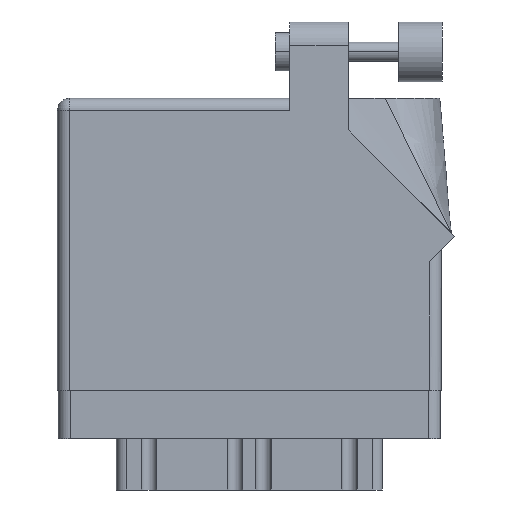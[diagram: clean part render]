
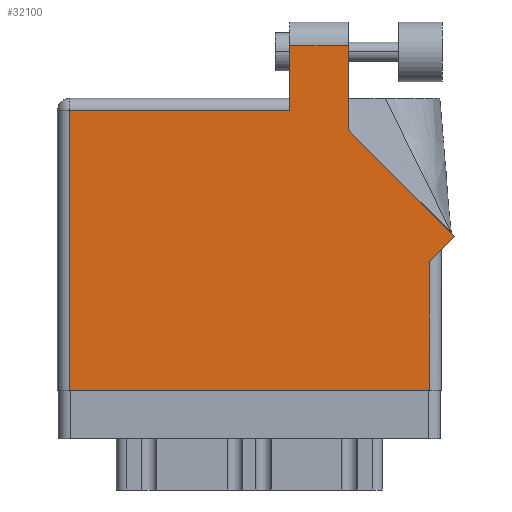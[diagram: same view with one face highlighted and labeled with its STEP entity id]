
A CAD part, front view. The second image highlights one B-rep face of the part: STEP entity #32100.
In plain terms, the highlighted face is planar.
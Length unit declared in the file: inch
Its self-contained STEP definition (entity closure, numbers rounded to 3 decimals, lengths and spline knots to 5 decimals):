
#353 = LINE ( 'NONE', #11561, #33160 ) ;
#774 = DIRECTION ( 'NONE',  ( -0.707, 0.707, 0. ) ) ;
#1603 = ORIENTED_EDGE ( 'NONE', *, *, #16011, .T. ) ;
#1677 = DIRECTION ( 'NONE',  ( 0., -1., 0. ) ) ;
#3643 = VECTOR ( 'NONE', #8445, 39.37008 ) ;
#3685 = DIRECTION ( 'NONE',  ( -1., 0., 0. ) ) ;
#4979 = LINE ( 'NONE', #26040, #32071 ) ;
#5489 = ORIENTED_EDGE ( 'NONE', *, *, #28860, .T. ) ;
#5757 = EDGE_CURVE ( 'NONE', #19924, #21574, #16168, .T. ) ;
#6481 = DIRECTION ( 'NONE',  ( 0., 0., -1. ) ) ;
#7013 = VERTEX_POINT ( 'NONE', #24255 ) ;
#7125 = ORIENTED_EDGE ( 'NONE', *, *, #5757, .T. ) ;
#7313 = VECTOR ( 'NONE', #7698, 39.37008 ) ;
#7698 = DIRECTION ( 'NONE',  ( 1., 0., 0. ) ) ;
#7923 = CARTESIAN_POINT ( 'NONE',  ( 0.062, 1.468, 0. ) ) ;
#8445 = DIRECTION ( 'NONE',  ( 0., 1., 0. ) ) ;
#10017 = ORIENTED_EDGE ( 'NONE', *, *, #15736, .T. ) ;
#11110 = CARTESIAN_POINT ( 'NONE',  ( 2.08071, 0.80771, 0. ) ) ;
#11286 = EDGE_CURVE ( 'NONE', #31697, #19924, #23322, .T. ) ;
#11561 = CARTESIAN_POINT ( 'NONE',  ( 1.217, 1.805, 0. ) ) ;
#11935 = CARTESIAN_POINT ( 'NONE',  ( 1.948, 0., 0. ) ) ;
#12372 = CARTESIAN_POINT ( 'NONE',  ( 2.01, 0.737, 0. ) ) ;
#12981 = VECTOR ( 'NONE', #1677, 39.37008 ) ;
#13047 = CARTESIAN_POINT ( 'NONE',  ( 1.524, 1.805, 0. ) ) ;
#13271 = VERTEX_POINT ( 'NONE', #7923 ) ;
#14476 = DIRECTION ( 'NONE',  ( 0.707, 0.707, 0. ) ) ;
#14502 = EDGE_CURVE ( 'NONE', #21574, #20996, #17464, .T. ) ;
#14668 = CARTESIAN_POINT ( 'NONE',  ( 1.217, 1.53, 0. ) ) ;
#15683 = DIRECTION ( 'NONE',  ( 0., 1., 0. ) ) ;
#15736 = EDGE_CURVE ( 'NONE', #21581, #17201, #22571, .T. ) ;
#16011 = EDGE_CURVE ( 'NONE', #20996, #7013, #32349, .T. ) ;
#16168 = LINE ( 'NONE', #24581, #3643 ) ;
#16589 = AXIS2_PLACEMENT_3D ( 'NONE', #27550, #6481, #27721 ) ;
#16829 = FACE_OUTER_BOUND ( 'NONE', #25756, .T. ) ;
#17201 = VERTEX_POINT ( 'NONE', #31759 ) ;
#17464 = LINE ( 'NONE', #12372, #32975 ) ;
#19005 = VECTOR ( 'NONE', #34609, 39.37008 ) ;
#19924 = VERTEX_POINT ( 'NONE', #11935 ) ;
#20282 = ORIENTED_EDGE ( 'NONE', *, *, #32624, .T. ) ;
#20996 = VERTEX_POINT ( 'NONE', #31602 ) ;
#21574 = VERTEX_POINT ( 'NONE', #23625 ) ;
#21581 = VERTEX_POINT ( 'NONE', #29242 ) ;
#21683 = VECTOR ( 'NONE', #22548, 39.37008 ) ;
#22548 = DIRECTION ( 'NONE',  ( -1., 0., 0. ) ) ;
#22571 = LINE ( 'NONE', #14668, #12981 ) ;
#23099 = ORIENTED_EDGE ( 'NONE', *, *, #11286, .T. ) ;
#23322 = LINE ( 'NONE', #33680, #7313 ) ;
#23625 = CARTESIAN_POINT ( 'NONE',  ( 1.948, 0.675, 0. ) ) ;
#24255 = CARTESIAN_POINT ( 'NONE',  ( 1.524, 1.36442, 0. ) ) ;
#24581 = CARTESIAN_POINT ( 'NONE',  ( 1.948, 0.737, 0. ) ) ;
#25250 = PLANE ( 'NONE',  #16589 ) ;
#25756 = EDGE_LOOP ( 'NONE', ( #27430, #5489, #10017, #20282, #26414, #23099, #7125, #32611, #1603 ) ) ;
#25865 = CARTESIAN_POINT ( 'NONE',  ( 0.062, 0., 0. ) ) ;
#26040 = CARTESIAN_POINT ( 'NONE',  ( 1.524, 1.36442, 0. ) ) ;
#26068 = EDGE_CURVE ( 'NONE', #7013, #31414, #4979, .T. ) ;
#26414 = ORIENTED_EDGE ( 'NONE', *, *, #34094, .T. ) ;
#27430 = ORIENTED_EDGE ( 'NONE', *, *, #26068, .T. ) ;
#27550 = CARTESIAN_POINT ( 'NONE',  ( 0., 1.53, 0. ) ) ;
#27721 = DIRECTION ( 'NONE',  ( -1., 0., 0. ) ) ;
#27796 = CARTESIAN_POINT ( 'NONE',  ( 0., 1.468, 0. ) ) ;
#28622 = CARTESIAN_POINT ( 'NONE',  ( 0.062, 0., 0. ) ) ;
#28860 = EDGE_CURVE ( 'NONE', #31414, #21581, #353, .T. ) ;
#29242 = CARTESIAN_POINT ( 'NONE',  ( 1.217, 1.805, 0. ) ) ;
#30940 = VECTOR ( 'NONE', #774, 39.37008 ) ;
#31414 = VERTEX_POINT ( 'NONE', #13047 ) ;
#31602 = CARTESIAN_POINT ( 'NONE',  ( 2.08071, 0.80771, 0. ) ) ;
#31697 = VERTEX_POINT ( 'NONE', #28622 ) ;
#31759 = CARTESIAN_POINT ( 'NONE',  ( 1.217, 1.468, 0. ) ) ;
#32071 = VECTOR ( 'NONE', #15683, 39.37008 ) ;
#32100 = ADVANCED_FACE ( 'NONE', ( #16829 ), #25250, .F. ) ;
#32349 = LINE ( 'NONE', #11110, #30940 ) ;
#32611 = ORIENTED_EDGE ( 'NONE', *, *, #14502, .T. ) ;
#32624 = EDGE_CURVE ( 'NONE', #17201, #13271, #33064, .T. ) ;
#32975 = VECTOR ( 'NONE', #14476, 39.37008 ) ;
#33064 = LINE ( 'NONE', #27796, #21683 ) ;
#33160 = VECTOR ( 'NONE', #3685, 39.37008 ) ;
#33680 = CARTESIAN_POINT ( 'NONE',  ( 0., 0., 0. ) ) ;
#33926 = LINE ( 'NONE', #25865, #19005 ) ;
#34094 = EDGE_CURVE ( 'NONE', #13271, #31697, #33926, .T. ) ;
#34609 = DIRECTION ( 'NONE',  ( 0., -1., 0. ) ) ;
